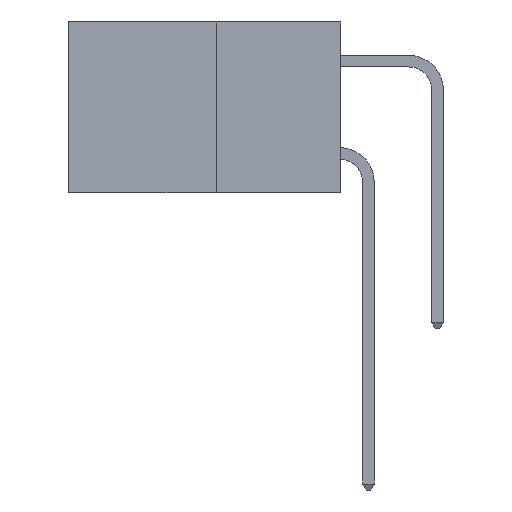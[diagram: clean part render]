
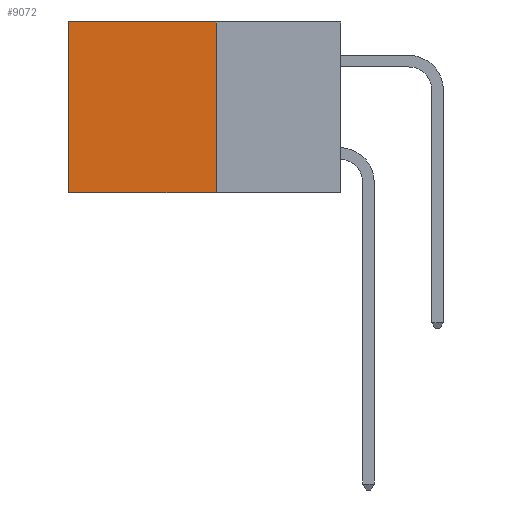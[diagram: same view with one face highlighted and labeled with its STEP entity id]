
A CAD part, left-side view. The second image highlights one B-rep face of the part: STEP entity #9072.
In plain terms, the highlighted planar face has unit normal (-1, 0, 0).
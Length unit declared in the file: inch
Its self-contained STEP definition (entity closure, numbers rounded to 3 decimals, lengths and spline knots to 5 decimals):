
#48 = VECTOR ( 'NONE', #4446, 39.37008 ) ;
#526 = LINE ( 'NONE', #21914, #33802 ) ;
#634 = DIRECTION ( 'NONE',  ( 0., 1., 0. ) ) ;
#1519 = PLANE ( 'NONE',  #19617 ) ;
#1746 = CARTESIAN_POINT ( 'NONE',  ( 0.277, 0.59, -0.37 ) ) ;
#2291 = CARTESIAN_POINT ( 'NONE',  ( 0.277, 0.59, -0.37 ) ) ;
#3895 = LINE ( 'NONE', #25022, #31008 ) ;
#4209 = DIRECTION ( 'NONE',  ( 0., 0., -1. ) ) ;
#4399 = EDGE_LOOP ( 'NONE', ( #13244, #17133, #28738, #23811 ) ) ;
#4446 = DIRECTION ( 'NONE',  ( 0., 0., -1. ) ) ;
#5202 = FACE_OUTER_BOUND ( 'NONE', #4399, .T. ) ;
#6250 = DIRECTION ( 'NONE',  ( 0., 0., -1. ) ) ;
#6634 = DIRECTION ( 'NONE',  ( 0., 1., 0. ) ) ;
#9072 = ADVANCED_FACE ( 'NONE', ( #5202 ), #1519, .F. ) ;
#11064 = EDGE_CURVE ( 'NONE', #19687, #25112, #20290, .T. ) ;
#11806 = VERTEX_POINT ( 'NONE', #33934 ) ;
#12195 = CARTESIAN_POINT ( 'NONE',  ( 0.277, 0.27, 0. ) ) ;
#13043 = LINE ( 'NONE', #13985, #20872 ) ;
#13244 = ORIENTED_EDGE ( 'NONE', *, *, #11064, .T. ) ;
#13985 = CARTESIAN_POINT ( 'NONE',  ( 0.277, 0.27, -0.37 ) ) ;
#14847 = EDGE_CURVE ( 'NONE', #26339, #19687, #3895, .T. ) ;
#15416 = EDGE_CURVE ( 'NONE', #26339, #11806, #526, .T. ) ;
#17133 = ORIENTED_EDGE ( 'NONE', *, *, #23388, .F. ) ;
#19617 = AXIS2_PLACEMENT_3D ( 'NONE', #30402, #20008, #4209 ) ;
#19687 = VERTEX_POINT ( 'NONE', #29423 ) ;
#20008 = DIRECTION ( 'NONE',  ( 1., 0., 0. ) ) ;
#20290 = LINE ( 'NONE', #1746, #48 ) ;
#20872 = VECTOR ( 'NONE', #634, 39.37008 ) ;
#21914 = CARTESIAN_POINT ( 'NONE',  ( 0.277, 0.27, -0.37 ) ) ;
#23388 = EDGE_CURVE ( 'NONE', #11806, #25112, #13043, .T. ) ;
#23811 = ORIENTED_EDGE ( 'NONE', *, *, #14847, .T. ) ;
#25022 = CARTESIAN_POINT ( 'NONE',  ( 0.277, 0.27, 0. ) ) ;
#25112 = VERTEX_POINT ( 'NONE', #2291 ) ;
#26339 = VERTEX_POINT ( 'NONE', #12195 ) ;
#28738 = ORIENTED_EDGE ( 'NONE', *, *, #15416, .F. ) ;
#29423 = CARTESIAN_POINT ( 'NONE',  ( 0.277, 0.59, 0. ) ) ;
#30402 = CARTESIAN_POINT ( 'NONE',  ( 0.277, 0.27, -0.37 ) ) ;
#31008 = VECTOR ( 'NONE', #6634, 39.37008 ) ;
#33802 = VECTOR ( 'NONE', #6250, 39.37008 ) ;
#33934 = CARTESIAN_POINT ( 'NONE',  ( 0.277, 0.27, -0.37 ) ) ;
